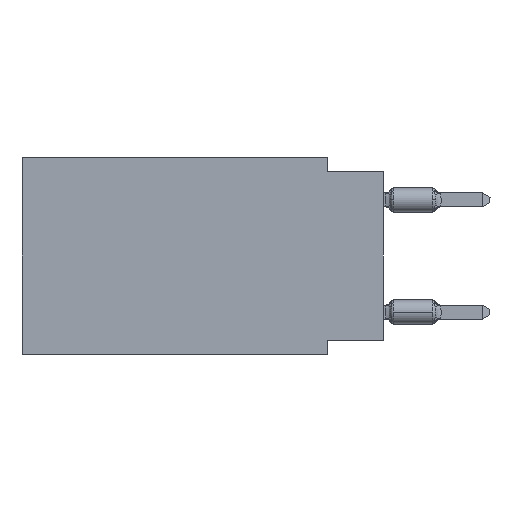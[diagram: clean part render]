
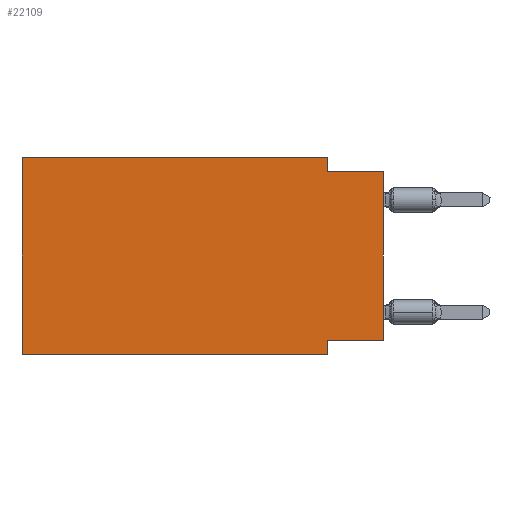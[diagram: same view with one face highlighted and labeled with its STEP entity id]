
A CAD part, left-side view. The second image highlights one B-rep face of the part: STEP entity #22109.
In plain terms, the highlighted planar face has unit normal (-1, 0, 0).
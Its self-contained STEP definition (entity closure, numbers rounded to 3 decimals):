
#195 = CARTESIAN_POINT ( 'NONE',  ( 0., 16.383, -8.89 ) ) ;
#253 = CARTESIAN_POINT ( 'NONE',  ( 0., 2.54, 0. ) ) ;
#626 = DIRECTION ( 'NONE',  ( 0., -1., 0. ) ) ;
#931 = FACE_OUTER_BOUND ( 'NONE', #40277, .T. ) ;
#1720 = CARTESIAN_POINT ( 'NONE',  ( 0., 16.383, -8.89 ) ) ;
#2056 = LINE ( 'NONE', #47476, #26145 ) ;
#2555 = EDGE_CURVE ( 'NONE', #44414, #8417, #2056, .T. ) ;
#2652 = CARTESIAN_POINT ( 'NONE',  ( 0., 0., -0.635 ) ) ;
#2781 = VERTEX_POINT ( 'NONE', #42002 ) ;
#3804 = LINE ( 'NONE', #27140, #22520 ) ;
#4405 = DIRECTION ( 'NONE',  ( 1., 0., 0. ) ) ;
#6193 = LINE ( 'NONE', #9669, #14623 ) ;
#6370 = ORIENTED_EDGE ( 'NONE', *, *, #40792, .F. ) ;
#6898 = VERTEX_POINT ( 'NONE', #10832 ) ;
#7940 = VECTOR ( 'NONE', #47864, 1000. ) ;
#8394 = LINE ( 'NONE', #35926, #45899 ) ;
#8417 = VERTEX_POINT ( 'NONE', #44319 ) ;
#9669 = CARTESIAN_POINT ( 'NONE',  ( 0., 2.54, -8.89 ) ) ;
#9912 = DIRECTION ( 'NONE',  ( 0., 0., -1. ) ) ;
#10832 = CARTESIAN_POINT ( 'NONE',  ( 0., 2.54, -8.255 ) ) ;
#11906 = VERTEX_POINT ( 'NONE', #13647 ) ;
#13265 = ORIENTED_EDGE ( 'NONE', *, *, #2555, .F. ) ;
#13647 = CARTESIAN_POINT ( 'NONE',  ( 0., 2.54, -8.89 ) ) ;
#13715 = DIRECTION ( 'NONE',  ( 0., 0., 1. ) ) ;
#14623 = VECTOR ( 'NONE', #9912, 1000. ) ;
#15034 = AXIS2_PLACEMENT_3D ( 'NONE', #27016, #4405, #43291 ) ;
#15076 = EDGE_CURVE ( 'NONE', #38540, #6898, #8394, .T. ) ;
#15186 = VECTOR ( 'NONE', #626, 1000. ) ;
#15255 = VERTEX_POINT ( 'NONE', #2652 ) ;
#16932 = ORIENTED_EDGE ( 'NONE', *, *, #24205, .F. ) ;
#17701 = CARTESIAN_POINT ( 'NONE',  ( 0., 0., -8.255 ) ) ;
#18783 = EDGE_CURVE ( 'NONE', #44414, #11906, #32746, .T. ) ;
#20337 = ORIENTED_EDGE ( 'NONE', *, *, #45379, .T. ) ;
#21989 = DIRECTION ( 'NONE',  ( 0., 0., -1. ) ) ;
#22109 = ADVANCED_FACE ( 'NONE', ( #931 ), #46998, .F. ) ;
#22520 = VECTOR ( 'NONE', #45000, 1000. ) ;
#22978 = LINE ( 'NONE', #34157, #15186 ) ;
#24205 = EDGE_CURVE ( 'NONE', #6898, #11906, #6193, .T. ) ;
#25081 = VERTEX_POINT ( 'NONE', #253 ) ;
#25716 = LINE ( 'NONE', #47799, #25746 ) ;
#25746 = VECTOR ( 'NONE', #21989, 1000. ) ;
#26145 = VECTOR ( 'NONE', #13715, 1000. ) ;
#27016 = CARTESIAN_POINT ( 'NONE',  ( 0., 16.383, 0. ) ) ;
#27127 = EDGE_CURVE ( 'NONE', #8417, #25081, #36171, .T. ) ;
#27140 = CARTESIAN_POINT ( 'NONE',  ( 0., 0., 0. ) ) ;
#28485 = CARTESIAN_POINT ( 'NONE',  ( 0., 16.383, 0. ) ) ;
#30313 = EDGE_CURVE ( 'NONE', #25081, #2781, #25716, .T. ) ;
#31166 = ORIENTED_EDGE ( 'NONE', *, *, #27127, .F. ) ;
#31186 = ORIENTED_EDGE ( 'NONE', *, *, #15076, .F. ) ;
#32207 = DIRECTION ( 'NONE',  ( 0., 1., 0. ) ) ;
#32746 = LINE ( 'NONE', #1720, #7940 ) ;
#34157 = CARTESIAN_POINT ( 'NONE',  ( 0., 0., -0.635 ) ) ;
#35812 = VECTOR ( 'NONE', #43634, 1000. ) ;
#35926 = CARTESIAN_POINT ( 'NONE',  ( 0., 0., -8.255 ) ) ;
#36171 = LINE ( 'NONE', #28485, #35812 ) ;
#37146 = ORIENTED_EDGE ( 'NONE', *, *, #18783, .T. ) ;
#37915 = ORIENTED_EDGE ( 'NONE', *, *, #30313, .F. ) ;
#38540 = VERTEX_POINT ( 'NONE', #17701 ) ;
#40277 = EDGE_LOOP ( 'NONE', ( #20337, #6370, #37915, #31166, #13265, #37146, #16932, #31186 ) ) ;
#40792 = EDGE_CURVE ( 'NONE', #2781, #15255, #22978, .T. ) ;
#42002 = CARTESIAN_POINT ( 'NONE',  ( 0., 2.54, -0.635 ) ) ;
#43291 = DIRECTION ( 'NONE',  ( 0., 0., -1. ) ) ;
#43634 = DIRECTION ( 'NONE',  ( 0., -1., 0. ) ) ;
#44319 = CARTESIAN_POINT ( 'NONE',  ( 0., 16.383, 0. ) ) ;
#44414 = VERTEX_POINT ( 'NONE', #195 ) ;
#45000 = DIRECTION ( 'NONE',  ( 0., 0., 1. ) ) ;
#45379 = EDGE_CURVE ( 'NONE', #38540, #15255, #3804, .T. ) ;
#45899 = VECTOR ( 'NONE', #32207, 1000. ) ;
#46998 = PLANE ( 'NONE',  #15034 ) ;
#47476 = CARTESIAN_POINT ( 'NONE',  ( 0., 16.383, 0. ) ) ;
#47799 = CARTESIAN_POINT ( 'NONE',  ( 0., 2.54, 0. ) ) ;
#47864 = DIRECTION ( 'NONE',  ( 0., -1., 0. ) ) ;
